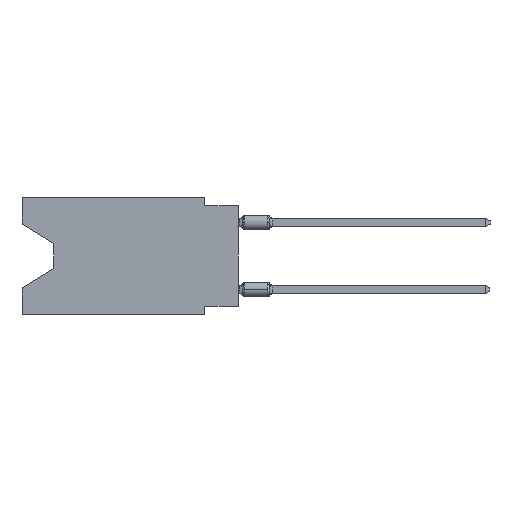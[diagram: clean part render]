
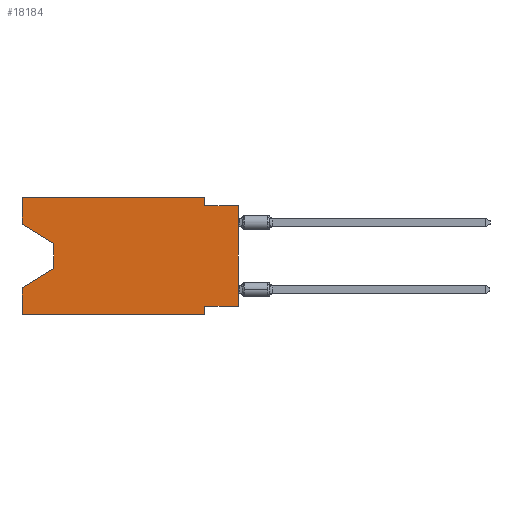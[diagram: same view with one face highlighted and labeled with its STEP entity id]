
A CAD part, left-side view. The second image highlights one B-rep face of the part: STEP entity #18184.
In plain terms, the highlighted planar face has unit normal (-1, 0, 0).
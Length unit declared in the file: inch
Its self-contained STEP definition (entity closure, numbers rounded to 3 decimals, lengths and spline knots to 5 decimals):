
#747 = CARTESIAN_POINT ( 'NONE',  ( 0., 0.645, -0.08025 ) ) ;
#2521 = VECTOR ( 'NONE', #33144, 39.37008 ) ;
#2624 = CARTESIAN_POINT ( 'NONE',  ( 0., 0.645, 0. ) ) ;
#3093 = VERTEX_POINT ( 'NONE', #27559 ) ;
#3584 = CARTESIAN_POINT ( 'NONE',  ( 0., 0.55, -0.212 ) ) ;
#4182 = EDGE_LOOP ( 'NONE', ( #16764, #12201, #27899, #25809, #30288, #24488, #20704, #6943, #13091, #12909, #42019, #40352 ) ) ;
#4664 = VERTEX_POINT ( 'NONE', #6122 ) ;
#5017 = LINE ( 'NONE', #25362, #34443 ) ;
#6122 = CARTESIAN_POINT ( 'NONE',  ( 0., 0.645, -0.35 ) ) ;
#6243 = CARTESIAN_POINT ( 'NONE',  ( 0., 0.1, -0.325 ) ) ;
#6603 = DIRECTION ( 'NONE',  ( 0., 0., -1. ) ) ;
#6724 = EDGE_CURVE ( 'NONE', #27215, #39684, #30132, .T. ) ;
#6943 = ORIENTED_EDGE ( 'NONE', *, *, #17983, .T. ) ;
#7582 = EDGE_CURVE ( 'NONE', #4664, #39684, #30021, .T. ) ;
#7731 = CARTESIAN_POINT ( 'NONE',  ( 0., 0.645, 0. ) ) ;
#7918 = EDGE_CURVE ( 'NONE', #4664, #19212, #5017, .T. ) ;
#8883 = VERTEX_POINT ( 'NONE', #24116 ) ;
#9076 = DIRECTION ( 'NONE',  ( 0., 0., 1. ) ) ;
#9682 = CARTESIAN_POINT ( 'NONE',  ( 0., 0., -0.325 ) ) ;
#9837 = LINE ( 'NONE', #27017, #10279 ) ;
#9957 = PLANE ( 'NONE',  #23613 ) ;
#10279 = VECTOR ( 'NONE', #40034, 39.37008 ) ;
#10747 = DIRECTION ( 'NONE',  ( 0., -1., 0. ) ) ;
#11126 = DIRECTION ( 'NONE',  ( 0., 0., -1. ) ) ;
#11189 = LINE ( 'NONE', #20698, #37342 ) ;
#11428 = CARTESIAN_POINT ( 'NONE',  ( 0., 0.1, 0. ) ) ;
#11579 = DIRECTION ( 'NONE',  ( 0., 0., 1. ) ) ;
#11962 = EDGE_CURVE ( 'NONE', #14984, #3093, #11189, .T. ) ;
#12201 = ORIENTED_EDGE ( 'NONE', *, *, #43529, .T. ) ;
#12839 = EDGE_CURVE ( 'NONE', #21675, #19212, #40831, .T. ) ;
#12909 = ORIENTED_EDGE ( 'NONE', *, *, #42137, .F. ) ;
#13091 = ORIENTED_EDGE ( 'NONE', *, *, #11962, .F. ) ;
#13358 = CARTESIAN_POINT ( 'NONE',  ( 0., 0.55, -0.212 ) ) ;
#13698 = CARTESIAN_POINT ( 'NONE',  ( 0., 0.1, -0.35 ) ) ;
#14439 = LINE ( 'NONE', #41347, #41224 ) ;
#14984 = VERTEX_POINT ( 'NONE', #24629 ) ;
#16764 = ORIENTED_EDGE ( 'NONE', *, *, #42163, .T. ) ;
#16770 = LINE ( 'NONE', #2624, #2521 ) ;
#17413 = VERTEX_POINT ( 'NONE', #11428 ) ;
#17983 = EDGE_CURVE ( 'NONE', #8883, #3093, #32919, .T. ) ;
#18080 = DIRECTION ( 'NONE',  ( 0., -1., 0. ) ) ;
#18184 = ADVANCED_FACE ( 'NONE', ( #30250 ), #9957, .F. ) ;
#18960 = EDGE_CURVE ( 'NONE', #21366, #17413, #24984, .T. ) ;
#19212 = VERTEX_POINT ( 'NONE', #39697 ) ;
#19920 = CARTESIAN_POINT ( 'NONE',  ( 0., 0.55, -0.138 ) ) ;
#19977 = LINE ( 'NONE', #33005, #41987 ) ;
#20048 = LINE ( 'NONE', #9682, #27843 ) ;
#20136 = DIRECTION ( 'NONE',  ( 0., 0., -1. ) ) ;
#20235 = VECTOR ( 'NONE', #9076, 39.37008 ) ;
#20698 = CARTESIAN_POINT ( 'NONE',  ( 0., 0., -0.025 ) ) ;
#20704 = ORIENTED_EDGE ( 'NONE', *, *, #34755, .F. ) ;
#21366 = VERTEX_POINT ( 'NONE', #34094 ) ;
#21675 = VERTEX_POINT ( 'NONE', #6243 ) ;
#22954 = DIRECTION ( 'NONE',  ( 0., 1., 0. ) ) ;
#23613 = AXIS2_PLACEMENT_3D ( 'NONE', #36864, #32903, #6603 ) ;
#24116 = CARTESIAN_POINT ( 'NONE',  ( 0., 0., -0.325 ) ) ;
#24312 = VERTEX_POINT ( 'NONE', #747 ) ;
#24488 = ORIENTED_EDGE ( 'NONE', *, *, #12839, .F. ) ;
#24629 = CARTESIAN_POINT ( 'NONE',  ( 0., 0.1, -0.025 ) ) ;
#24984 = LINE ( 'NONE', #7731, #34839 ) ;
#25362 = CARTESIAN_POINT ( 'NONE',  ( 0., 0.645, -0.35 ) ) ;
#25809 = ORIENTED_EDGE ( 'NONE', *, *, #7582, .F. ) ;
#27017 = CARTESIAN_POINT ( 'NONE',  ( 0., 0.645, -0.08025 ) ) ;
#27215 = VERTEX_POINT ( 'NONE', #13358 ) ;
#27559 = CARTESIAN_POINT ( 'NONE',  ( 0., 0., -0.025 ) ) ;
#27843 = VECTOR ( 'NONE', #22954, 39.37008 ) ;
#27899 = ORIENTED_EDGE ( 'NONE', *, *, #6724, .T. ) ;
#28575 = CARTESIAN_POINT ( 'NONE',  ( 0., 0., 0. ) ) ;
#29240 = VECTOR ( 'NONE', #11579, 39.37008 ) ;
#30021 = LINE ( 'NONE', #36637, #20235 ) ;
#30132 = LINE ( 'NONE', #3584, #41299 ) ;
#30250 = FACE_OUTER_BOUND ( 'NONE', #4182, .T. ) ;
#30288 = ORIENTED_EDGE ( 'NONE', *, *, #7918, .T. ) ;
#32282 = CARTESIAN_POINT ( 'NONE',  ( 0., 0.645, -0.26975 ) ) ;
#32477 = VECTOR ( 'NONE', #20136, 39.37008 ) ;
#32903 = DIRECTION ( 'NONE',  ( 1., 0., 0. ) ) ;
#32919 = LINE ( 'NONE', #28575, #29240 ) ;
#33005 = CARTESIAN_POINT ( 'NONE',  ( 0., 0.1, 0. ) ) ;
#33144 = DIRECTION ( 'NONE',  ( 0., 0., 1. ) ) ;
#34094 = CARTESIAN_POINT ( 'NONE',  ( 0., 0.645, 0. ) ) ;
#34205 = VERTEX_POINT ( 'NONE', #19920 ) ;
#34443 = VECTOR ( 'NONE', #18080, 39.37008 ) ;
#34674 = DIRECTION ( 'NONE',  ( 0., -1., 0. ) ) ;
#34755 = EDGE_CURVE ( 'NONE', #8883, #21675, #20048, .T. ) ;
#34839 = VECTOR ( 'NONE', #34674, 39.37008 ) ;
#36314 = DIRECTION ( 'NONE',  ( 0., 0., -1. ) ) ;
#36637 = CARTESIAN_POINT ( 'NONE',  ( 0., 0.645, 0. ) ) ;
#36864 = CARTESIAN_POINT ( 'NONE',  ( 0., 0.645, 0. ) ) ;
#37342 = VECTOR ( 'NONE', #10747, 39.37008 ) ;
#39684 = VERTEX_POINT ( 'NONE', #32282 ) ;
#39697 = CARTESIAN_POINT ( 'NONE',  ( 0., 0.1, -0.35 ) ) ;
#40034 = DIRECTION ( 'NONE',  ( 0., -0.855, -0.519 ) ) ;
#40040 = DIRECTION ( 'NONE',  ( 0., 0.855, -0.519 ) ) ;
#40352 = ORIENTED_EDGE ( 'NONE', *, *, #40775, .F. ) ;
#40775 = EDGE_CURVE ( 'NONE', #24312, #21366, #16770, .T. ) ;
#40831 = LINE ( 'NONE', #13698, #32477 ) ;
#41224 = VECTOR ( 'NONE', #11126, 39.37008 ) ;
#41299 = VECTOR ( 'NONE', #40040, 39.37008 ) ;
#41347 = CARTESIAN_POINT ( 'NONE',  ( 0., 0.55, -0.138 ) ) ;
#41987 = VECTOR ( 'NONE', #36314, 39.37008 ) ;
#42019 = ORIENTED_EDGE ( 'NONE', *, *, #18960, .F. ) ;
#42137 = EDGE_CURVE ( 'NONE', #17413, #14984, #19977, .T. ) ;
#42163 = EDGE_CURVE ( 'NONE', #24312, #34205, #9837, .T. ) ;
#43529 = EDGE_CURVE ( 'NONE', #34205, #27215, #14439, .T. ) ;
